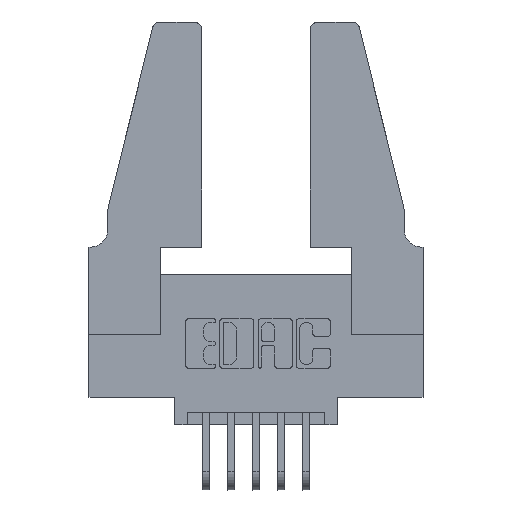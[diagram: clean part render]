
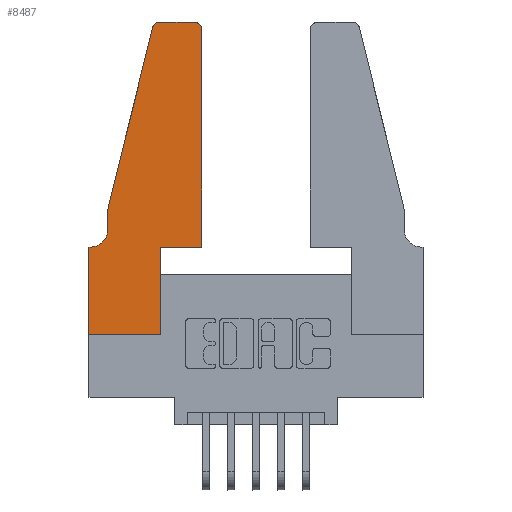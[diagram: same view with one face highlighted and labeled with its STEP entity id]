
A CAD part, top view. The second image highlights one B-rep face of the part: STEP entity #8487.
In plain terms, the highlighted planar face has unit normal (0, 0, 1).
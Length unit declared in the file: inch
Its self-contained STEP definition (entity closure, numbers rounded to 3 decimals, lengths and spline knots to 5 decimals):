
#106 = DIRECTION ( 'NONE',  ( 1., 0., 0. ) ) ;
#151 = CARTESIAN_POINT ( 'NONE',  ( 0., 0., 0.37 ) ) ;
#153 = CARTESIAN_POINT ( 'NONE',  ( 0.0755, 0.35, 0.37 ) ) ;
#157 = EDGE_CURVE ( 'NONE', #5046, #11140, #361, .T. ) ;
#361 = LINE ( 'NONE', #7392, #9212 ) ;
#491 = DIRECTION ( 'NONE',  ( -0.239, -0.971, 0. ) ) ;
#548 = ORIENTED_EDGE ( 'NONE', *, *, #157, .T. ) ;
#593 = DIRECTION ( 'NONE',  ( 0., 0., -1. ) ) ;
#617 = ORIENTED_EDGE ( 'NONE', *, *, #9858, .T. ) ;
#680 = DIRECTION ( 'NONE',  ( 1., 0., 0. ) ) ;
#776 = EDGE_CURVE ( 'NONE', #6238, #7097, #3676, .T. ) ;
#858 = DIRECTION ( 'NONE',  ( 0., -1., 0. ) ) ;
#903 = CARTESIAN_POINT ( 'NONE',  ( 0.284, 1.22, 0.37 ) ) ;
#973 = CARTESIAN_POINT ( 'NONE',  ( 0.4505, 0.35, 0.37 ) ) ;
#1139 = AXIS2_PLACEMENT_3D ( 'NONE', #8587, #3560, #9450 ) ;
#1342 = VECTOR ( 'NONE', #7649, 39.37008 ) ;
#1350 = LINE ( 'NONE', #973, #10130 ) ;
#1389 = AXIS2_PLACEMENT_3D ( 'NONE', #5807, #593, #6629 ) ;
#1422 = ORIENTED_EDGE ( 'NONE', *, *, #7093, .T. ) ;
#1430 = CARTESIAN_POINT ( 'NONE',  ( 0.0755, 0.5, 0.37 ) ) ;
#1550 = VERTEX_POINT ( 'NONE', #3093 ) ;
#1838 = DIRECTION ( 'NONE',  ( 1., 0., 0. ) ) ;
#1867 = CIRCLE ( 'NONE', #10590, 0.03 ) ;
#1918 = CARTESIAN_POINT ( 'NONE',  ( 0., 0., 0.37 ) ) ;
#1949 = VERTEX_POINT ( 'NONE', #2918 ) ;
#2154 = CARTESIAN_POINT ( 'NONE',  ( 0., 0., 0.37 ) ) ;
#2163 = VERTEX_POINT ( 'NONE', #5567 ) ;
#2399 = CARTESIAN_POINT ( 'NONE',  ( 0.0055, 0.35, 0.37 ) ) ;
#2522 = LINE ( 'NONE', #8496, #6501 ) ;
#2691 = PLANE ( 'NONE',  #1139 ) ;
#2918 = CARTESIAN_POINT ( 'NONE',  ( 0., 0.35, 0.37 ) ) ;
#2989 = EDGE_CURVE ( 'NONE', #1550, #8278, #3133, .T. ) ;
#3093 = CARTESIAN_POINT ( 'NONE',  ( 0.0755, 0.42, 0.37 ) ) ;
#3133 = CIRCLE ( 'NONE', #1389, 0.07 ) ;
#3426 = ORIENTED_EDGE ( 'NONE', *, *, #3854, .T. ) ;
#3524 = CARTESIAN_POINT ( 'NONE',  ( 0.284, 1.25, 0.37 ) ) ;
#3560 = DIRECTION ( 'NONE',  ( 0., 0., 1. ) ) ;
#3625 = DIRECTION ( 'NONE',  ( 0., 1., 0. ) ) ;
#3676 = LINE ( 'NONE', #151, #3946 ) ;
#3718 = DIRECTION ( 'NONE',  ( 1., 0., 0. ) ) ;
#3854 = EDGE_CURVE ( 'NONE', #7223, #8815, #1350, .T. ) ;
#3926 = LINE ( 'NONE', #5950, #1342 ) ;
#3943 = CARTESIAN_POINT ( 'NONE',  ( 0.4205, 1.25, 0.37 ) ) ;
#3946 = VECTOR ( 'NONE', #106, 39.37008 ) ;
#4328 = ORIENTED_EDGE ( 'NONE', *, *, #4522, .T. ) ;
#4522 = EDGE_CURVE ( 'NONE', #8278, #1949, #10249, .T. ) ;
#4678 = ORIENTED_EDGE ( 'NONE', *, *, #2989, .T. ) ;
#4975 = EDGE_CURVE ( 'NONE', #7097, #2163, #3926, .T. ) ;
#5046 = VERTEX_POINT ( 'NONE', #3943 ) ;
#5171 = ORIENTED_EDGE ( 'NONE', *, *, #4975, .T. ) ;
#5240 = CARTESIAN_POINT ( 'NONE',  ( 0.2865, 0., 0.37 ) ) ;
#5567 = CARTESIAN_POINT ( 'NONE',  ( 0.2865, 0.35, 0.37 ) ) ;
#5722 = EDGE_CURVE ( 'NONE', #7642, #9157, #7449, .T. ) ;
#5807 = CARTESIAN_POINT ( 'NONE',  ( 0.0055, 0.42, 0.37 ) ) ;
#5881 = DIRECTION ( 'NONE',  ( 0., 0., 1. ) ) ;
#5905 = DIRECTION ( 'NONE',  ( -1., 0., 0. ) ) ;
#5950 = CARTESIAN_POINT ( 'NONE',  ( 0.2865, 0.35, 0.37 ) ) ;
#6238 = VERTEX_POINT ( 'NONE', #2154 ) ;
#6430 = ORIENTED_EDGE ( 'NONE', *, *, #776, .T. ) ;
#6476 = EDGE_CURVE ( 'NONE', #8815, #5046, #8204, .T. ) ;
#6501 = VECTOR ( 'NONE', #858, 39.37008 ) ;
#6629 = DIRECTION ( 'NONE',  ( -1., 0., 0. ) ) ;
#6682 = CARTESIAN_POINT ( 'NONE',  ( 0.25487, 1.22718, 0.37 ) ) ;
#6905 = DIRECTION ( 'NONE',  ( 0., 0., 1. ) ) ;
#6945 = FACE_OUTER_BOUND ( 'NONE', #8322, .T. ) ;
#7040 = CARTESIAN_POINT ( 'NONE',  ( 0.4505, 0.35, 0.37 ) ) ;
#7046 = CARTESIAN_POINT ( 'NONE',  ( 0.4505, 0.35, 0.37 ) ) ;
#7093 = EDGE_CURVE ( 'NONE', #11140, #7642, #1867, .T. ) ;
#7097 = VERTEX_POINT ( 'NONE', #5240 ) ;
#7223 = VERTEX_POINT ( 'NONE', #7040 ) ;
#7368 = VECTOR ( 'NONE', #3718, 39.37008 ) ;
#7392 = CARTESIAN_POINT ( 'NONE',  ( 0.2605, 1.25, 0.37 ) ) ;
#7449 = LINE ( 'NONE', #1430, #9431 ) ;
#7610 = AXIS2_PLACEMENT_3D ( 'NONE', #10909, #5881, #680 ) ;
#7642 = VERTEX_POINT ( 'NONE', #6682 ) ;
#7649 = DIRECTION ( 'NONE',  ( 0., 1., 0. ) ) ;
#7718 = EDGE_CURVE ( 'NONE', #9157, #1550, #2522, .T. ) ;
#7821 = DIRECTION ( 'NONE',  ( 0., -1., 0. ) ) ;
#8076 = ORIENTED_EDGE ( 'NONE', *, *, #9795, .T. ) ;
#8146 = VECTOR ( 'NONE', #7821, 39.37008 ) ;
#8184 = ORIENTED_EDGE ( 'NONE', *, *, #7718, .T. ) ;
#8204 = CIRCLE ( 'NONE', #7610, 0.03 ) ;
#8278 = VERTEX_POINT ( 'NONE', #2399 ) ;
#8322 = EDGE_LOOP ( 'NONE', ( #548, #1422, #9046, #8184, #4678, #4328, #8076, #6430, #5171, #617, #3426, #10950 ) ) ;
#8487 = ADVANCED_FACE ( 'NONE', ( #6945 ), #2691, .T. ) ;
#8496 = CARTESIAN_POINT ( 'NONE',  ( 0.0755, 0.5, 0.37 ) ) ;
#8587 = CARTESIAN_POINT ( 'NONE',  ( 0., 0.35, 0.37 ) ) ;
#8602 = CARTESIAN_POINT ( 'NONE',  ( 0.0755, 0.5, 0.37 ) ) ;
#8745 = DIRECTION ( 'NONE',  ( -1., 0., 0. ) ) ;
#8815 = VERTEX_POINT ( 'NONE', #10665 ) ;
#9046 = ORIENTED_EDGE ( 'NONE', *, *, #5722, .T. ) ;
#9157 = VERTEX_POINT ( 'NONE', #8602 ) ;
#9212 = VECTOR ( 'NONE', #5905, 39.37008 ) ;
#9431 = VECTOR ( 'NONE', #491, 39.37008 ) ;
#9450 = DIRECTION ( 'NONE',  ( 1., 0., 0. ) ) ;
#9608 = LINE ( 'NONE', #7046, #7368 ) ;
#9795 = EDGE_CURVE ( 'NONE', #1949, #6238, #10413, .T. ) ;
#9858 = EDGE_CURVE ( 'NONE', #2163, #7223, #9608, .T. ) ;
#9980 = VECTOR ( 'NONE', #8745, 39.37008 ) ;
#10130 = VECTOR ( 'NONE', #3625, 39.37008 ) ;
#10249 = LINE ( 'NONE', #153, #9980 ) ;
#10413 = LINE ( 'NONE', #1918, #8146 ) ;
#10590 = AXIS2_PLACEMENT_3D ( 'NONE', #903, #6905, #1838 ) ;
#10665 = CARTESIAN_POINT ( 'NONE',  ( 0.4505, 1.22, 0.37 ) ) ;
#10909 = CARTESIAN_POINT ( 'NONE',  ( 0.4205, 1.22, 0.37 ) ) ;
#10950 = ORIENTED_EDGE ( 'NONE', *, *, #6476, .T. ) ;
#11140 = VERTEX_POINT ( 'NONE', #3524 ) ;
